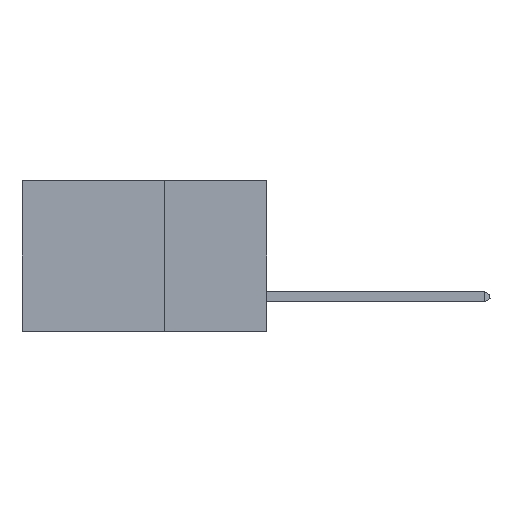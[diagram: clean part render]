
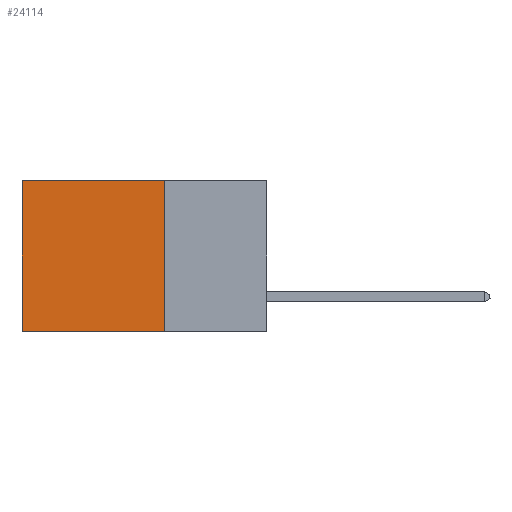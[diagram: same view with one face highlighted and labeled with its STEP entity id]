
A CAD part, left-side view. The second image highlights one B-rep face of the part: STEP entity #24114.
In plain terms, the highlighted planar face has unit normal (-1, 0, 0).
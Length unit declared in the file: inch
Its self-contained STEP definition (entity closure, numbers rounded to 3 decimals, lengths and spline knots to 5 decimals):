
#336 = CARTESIAN_POINT ( 'NONE',  ( 0.2875, 0.25, -0.37 ) ) ;
#2947 = AXIS2_PLACEMENT_3D ( 'NONE', #26292, #32210, #14212 ) ;
#3436 = CARTESIAN_POINT ( 'NONE',  ( 0.2875, 0.6, 0. ) ) ;
#5332 = VECTOR ( 'NONE', #18443, 39.37008 ) ;
#8116 = PLANE ( 'NONE',  #2947 ) ;
#8401 = ORIENTED_EDGE ( 'NONE', *, *, #9049, .T. ) ;
#9049 = EDGE_CURVE ( 'NONE', #30584, #38095, #27203, .T. ) ;
#9671 = CARTESIAN_POINT ( 'NONE',  ( 0.2875, 0.25, 0. ) ) ;
#11237 = ORIENTED_EDGE ( 'NONE', *, *, #31087, .T. ) ;
#13218 = EDGE_LOOP ( 'NONE', ( #11237, #30941, #35171, #8401 ) ) ;
#14212 = DIRECTION ( 'NONE',  ( 0., 0., -1. ) ) ;
#16783 = CARTESIAN_POINT ( 'NONE',  ( 0.2875, 0.25, 0. ) ) ;
#18443 = DIRECTION ( 'NONE',  ( 0., 1., 0. ) ) ;
#18492 = VERTEX_POINT ( 'NONE', #33930 ) ;
#18929 = DIRECTION ( 'NONE',  ( 0., 0., -1. ) ) ;
#20437 = VERTEX_POINT ( 'NONE', #29649 ) ;
#20891 = LINE ( 'NONE', #9671, #36424 ) ;
#21395 = EDGE_CURVE ( 'NONE', #18492, #20437, #25126, .T. ) ;
#23517 = VECTOR ( 'NONE', #33457, 39.37008 ) ;
#24007 = CARTESIAN_POINT ( 'NONE',  ( 0.2875, 0.25, 0. ) ) ;
#24114 = ADVANCED_FACE ( 'NONE', ( #37553 ), #8116, .F. ) ;
#25126 = LINE ( 'NONE', #336, #5332 ) ;
#26061 = CARTESIAN_POINT ( 'NONE',  ( 0.2875, 0.6, 0. ) ) ;
#26292 = CARTESIAN_POINT ( 'NONE',  ( 0.2875, 0.25, 0. ) ) ;
#27203 = LINE ( 'NONE', #24007, #37101 ) ;
#27856 = EDGE_CURVE ( 'NONE', #30584, #18492, #20891, .T. ) ;
#29649 = CARTESIAN_POINT ( 'NONE',  ( 0.2875, 0.6, -0.37 ) ) ;
#30584 = VERTEX_POINT ( 'NONE', #16783 ) ;
#30941 = ORIENTED_EDGE ( 'NONE', *, *, #21395, .F. ) ;
#31087 = EDGE_CURVE ( 'NONE', #38095, #20437, #32427, .T. ) ;
#31601 = DIRECTION ( 'NONE',  ( 0., 1., 0. ) ) ;
#32210 = DIRECTION ( 'NONE',  ( 1., 0., 0. ) ) ;
#32427 = LINE ( 'NONE', #3436, #23517 ) ;
#33457 = DIRECTION ( 'NONE',  ( 0., 0., -1. ) ) ;
#33930 = CARTESIAN_POINT ( 'NONE',  ( 0.2875, 0.25, -0.37 ) ) ;
#35171 = ORIENTED_EDGE ( 'NONE', *, *, #27856, .F. ) ;
#36424 = VECTOR ( 'NONE', #18929, 39.37008 ) ;
#37101 = VECTOR ( 'NONE', #31601, 39.37008 ) ;
#37553 = FACE_OUTER_BOUND ( 'NONE', #13218, .T. ) ;
#38095 = VERTEX_POINT ( 'NONE', #26061 ) ;
